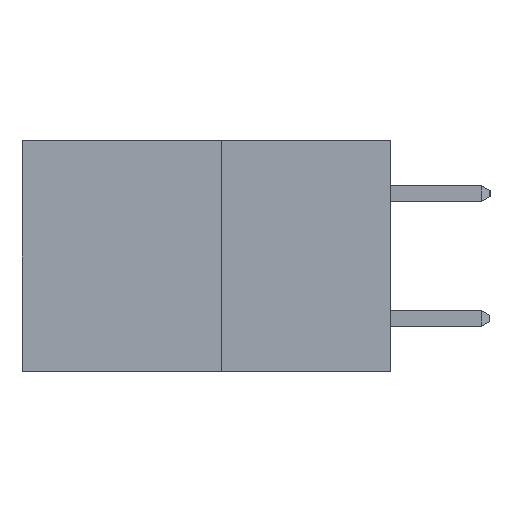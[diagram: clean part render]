
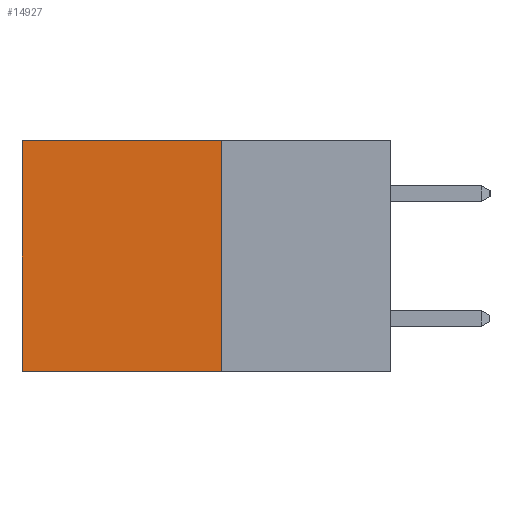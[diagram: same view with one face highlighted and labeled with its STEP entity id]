
A CAD part, left-side view. The second image highlights one B-rep face of the part: STEP entity #14927.
In plain terms, the highlighted planar face has unit normal (-1, 0, 0).
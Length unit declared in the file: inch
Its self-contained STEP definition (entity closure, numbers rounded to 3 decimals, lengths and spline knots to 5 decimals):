
#113 = LINE ( 'NONE', #8266, #14115 ) ;
#1104 = CARTESIAN_POINT ( 'NONE',  ( 0.277, 0.27, -0.37 ) ) ;
#1216 = EDGE_CURVE ( 'NONE', #12016, #11622, #113, .T. ) ;
#1650 = EDGE_CURVE ( 'NONE', #11030, #7794, #10396, .T. ) ;
#1796 = FACE_OUTER_BOUND ( 'NONE', #9627, .T. ) ;
#2944 = DIRECTION ( 'NONE',  ( 0., 0., -1. ) ) ;
#3207 = LINE ( 'NONE', #22493, #21968 ) ;
#3504 = CARTESIAN_POINT ( 'NONE',  ( 0.277, 0.27, 0. ) ) ;
#3600 = EDGE_CURVE ( 'NONE', #11030, #12016, #14231, .T. ) ;
#3692 = AXIS2_PLACEMENT_3D ( 'NONE', #1104, #13877, #2944 ) ;
#7794 = VERTEX_POINT ( 'NONE', #11302 ) ;
#7869 = CARTESIAN_POINT ( 'NONE',  ( 0.277, 0.27, -0.37 ) ) ;
#7943 = DIRECTION ( 'NONE',  ( 0., 0., -1. ) ) ;
#7958 = EDGE_CURVE ( 'NONE', #7794, #11622, #3207, .T. ) ;
#8216 = DIRECTION ( 'NONE',  ( 0., 1., 0. ) ) ;
#8266 = CARTESIAN_POINT ( 'NONE',  ( 0.277, 0.27, -0.37 ) ) ;
#9157 = ORIENTED_EDGE ( 'NONE', *, *, #1650, .T. ) ;
#9619 = CARTESIAN_POINT ( 'NONE',  ( 0.277, 0.27, -0.37 ) ) ;
#9627 = EDGE_LOOP ( 'NONE', ( #21014, #23169, #23299, #9157 ) ) ;
#9836 = VECTOR ( 'NONE', #21051, 39.37008 ) ;
#10396 = LINE ( 'NONE', #15850, #9836 ) ;
#11030 = VERTEX_POINT ( 'NONE', #3504 ) ;
#11302 = CARTESIAN_POINT ( 'NONE',  ( 0.277, 0.59, 0. ) ) ;
#11622 = VERTEX_POINT ( 'NONE', #15842 ) ;
#12016 = VERTEX_POINT ( 'NONE', #9619 ) ;
#13659 = VECTOR ( 'NONE', #7943, 39.37008 ) ;
#13877 = DIRECTION ( 'NONE',  ( 1., 0., 0. ) ) ;
#14115 = VECTOR ( 'NONE', #8216, 39.37008 ) ;
#14231 = LINE ( 'NONE', #7869, #13659 ) ;
#14927 = ADVANCED_FACE ( 'NONE', ( #1796 ), #22848, .F. ) ;
#15360 = DIRECTION ( 'NONE',  ( 0., 0., -1. ) ) ;
#15842 = CARTESIAN_POINT ( 'NONE',  ( 0.277, 0.59, -0.37 ) ) ;
#15850 = CARTESIAN_POINT ( 'NONE',  ( 0.277, 0.27, 0. ) ) ;
#21014 = ORIENTED_EDGE ( 'NONE', *, *, #7958, .T. ) ;
#21051 = DIRECTION ( 'NONE',  ( 0., 1., 0. ) ) ;
#21968 = VECTOR ( 'NONE', #15360, 39.37008 ) ;
#22493 = CARTESIAN_POINT ( 'NONE',  ( 0.277, 0.59, -0.37 ) ) ;
#22848 = PLANE ( 'NONE',  #3692 ) ;
#23169 = ORIENTED_EDGE ( 'NONE', *, *, #1216, .F. ) ;
#23299 = ORIENTED_EDGE ( 'NONE', *, *, #3600, .F. ) ;
